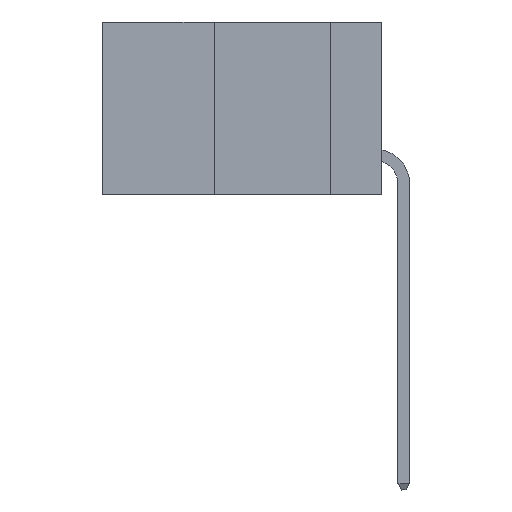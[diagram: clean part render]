
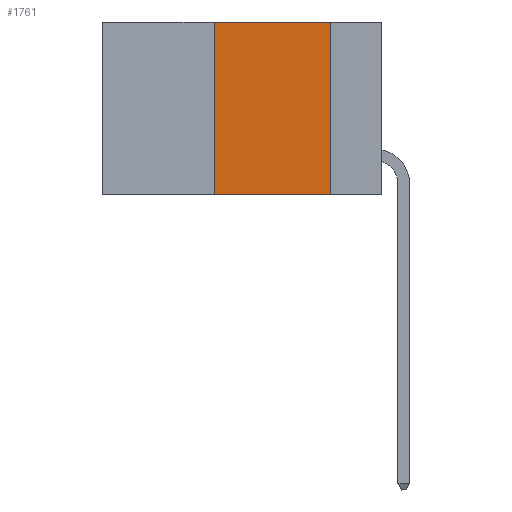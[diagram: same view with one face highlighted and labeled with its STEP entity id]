
A CAD part, left-side view. The second image highlights one B-rep face of the part: STEP entity #1761.
In plain terms, the highlighted planar face has unit normal (-1, 0, 0).
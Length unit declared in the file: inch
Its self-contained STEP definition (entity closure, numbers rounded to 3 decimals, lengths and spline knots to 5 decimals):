
#941 = EDGE_CURVE ( 'NONE', #36105, #9647, #27227, .T. ) ;
#1321 = AXIS2_PLACEMENT_3D ( 'NONE', #29377, #19695, #26319 ) ;
#1761 = ADVANCED_FACE ( 'NONE', ( #17333 ), #36482, .F. ) ;
#2544 = EDGE_CURVE ( 'NONE', #15194, #8511, #3305, .T. ) ;
#3305 = LINE ( 'NONE', #10469, #38529 ) ;
#3695 = ORIENTED_EDGE ( 'NONE', *, *, #31613, .F. ) ;
#5695 = ORIENTED_EDGE ( 'NONE', *, *, #941, .F. ) ;
#6079 = DIRECTION ( 'NONE',  ( 0., -1., 0. ) ) ;
#7756 = CARTESIAN_POINT ( 'NONE',  ( 0., 0.36, 0. ) ) ;
#8511 = VERTEX_POINT ( 'NONE', #27289 ) ;
#9647 = VERTEX_POINT ( 'NONE', #9668 ) ;
#9668 = CARTESIAN_POINT ( 'NONE',  ( 0., 0.36, 0. ) ) ;
#10469 = CARTESIAN_POINT ( 'NONE',  ( 0., 0.11, 0. ) ) ;
#10664 = DIRECTION ( 'NONE',  ( 0., 0., 1. ) ) ;
#11140 = CARTESIAN_POINT ( 'NONE',  ( 0., 0.36, -0.37 ) ) ;
#14009 = ORIENTED_EDGE ( 'NONE', *, *, #33510, .T. ) ;
#15194 = VERTEX_POINT ( 'NONE', #29849 ) ;
#17120 = DIRECTION ( 'NONE',  ( 0., 0., -1. ) ) ;
#17333 = FACE_OUTER_BOUND ( 'NONE', #35240, .T. ) ;
#19695 = DIRECTION ( 'NONE',  ( 1., 0., 0. ) ) ;
#21496 = CARTESIAN_POINT ( 'NONE',  ( 0., 0.6, -0.37 ) ) ;
#23022 = LINE ( 'NONE', #23120, #35460 ) ;
#23120 = CARTESIAN_POINT ( 'NONE',  ( 0., 0.6, 0. ) ) ;
#24652 = ORIENTED_EDGE ( 'NONE', *, *, #2544, .F. ) ;
#24978 = VECTOR ( 'NONE', #28408, 39.37008 ) ;
#26319 = DIRECTION ( 'NONE',  ( 0., 0., -1. ) ) ;
#27227 = LINE ( 'NONE', #7756, #36090 ) ;
#27289 = CARTESIAN_POINT ( 'NONE',  ( 0., 0.11, -0.37 ) ) ;
#28408 = DIRECTION ( 'NONE',  ( 0., -1., 0. ) ) ;
#29377 = CARTESIAN_POINT ( 'NONE',  ( 0., 0.6, 0. ) ) ;
#29849 = CARTESIAN_POINT ( 'NONE',  ( 0., 0.11, 0. ) ) ;
#31613 = EDGE_CURVE ( 'NONE', #9647, #15194, #23022, .T. ) ;
#33510 = EDGE_CURVE ( 'NONE', #36105, #8511, #39994, .T. ) ;
#35240 = EDGE_LOOP ( 'NONE', ( #24652, #3695, #5695, #14009 ) ) ;
#35460 = VECTOR ( 'NONE', #6079, 39.37008 ) ;
#36090 = VECTOR ( 'NONE', #10664, 39.37008 ) ;
#36105 = VERTEX_POINT ( 'NONE', #11140 ) ;
#36482 = PLANE ( 'NONE',  #1321 ) ;
#38529 = VECTOR ( 'NONE', #17120, 39.37008 ) ;
#39994 = LINE ( 'NONE', #21496, #24978 ) ;
